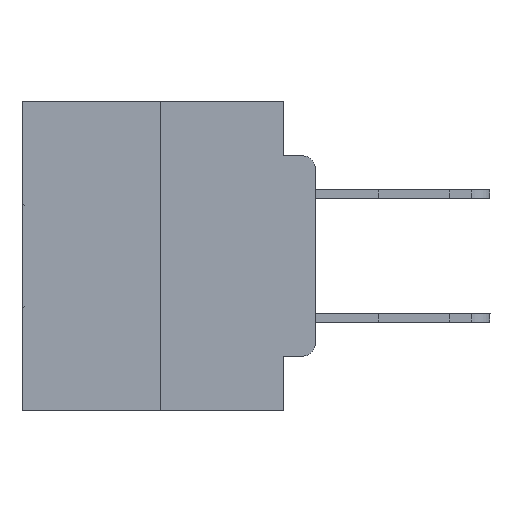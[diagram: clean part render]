
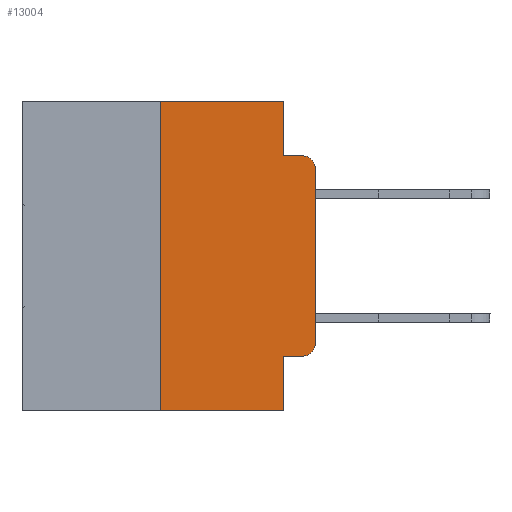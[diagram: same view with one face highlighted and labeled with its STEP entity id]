
A CAD part, left-side view. The second image highlights one B-rep face of the part: STEP entity #13004.
In plain terms, the highlighted planar face has unit normal (-1, 0, 0).
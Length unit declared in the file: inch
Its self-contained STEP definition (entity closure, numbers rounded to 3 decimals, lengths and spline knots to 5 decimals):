
#604 = EDGE_CURVE ( 'NONE', #9480, #17021, #27787, .T. ) ;
#773 = DIRECTION ( 'NONE',  ( 0., -1., 0. ) ) ;
#1050 = VERTEX_POINT ( 'NONE', #23095 ) ;
#1569 = ORIENTED_EDGE ( 'NONE', *, *, #604, .F. ) ;
#1609 = VECTOR ( 'NONE', #773, 39.37008 ) ;
#2639 = DIRECTION ( 'NONE',  ( 0., 0., -1. ) ) ;
#2685 = VECTOR ( 'NONE', #3333, 39.37008 ) ;
#3333 = DIRECTION ( 'NONE',  ( 0., 0., -1. ) ) ;
#3378 = CIRCLE ( 'NONE', #3551, 0.02 ) ;
#3551 = AXIS2_PLACEMENT_3D ( 'NONE', #14198, #12220, #28880 ) ;
#5192 = LINE ( 'NONE', #18729, #28688 ) ;
#5679 = DIRECTION ( 'NONE',  ( -1., 0., 0. ) ) ;
#5706 = CARTESIAN_POINT ( 'NONE',  ( 0., 0.051, 0. ) ) ;
#6138 = EDGE_CURVE ( 'NONE', #16923, #23357, #5192, .T. ) ;
#6221 = EDGE_CURVE ( 'NONE', #16923, #28515, #27536, .T. ) ;
#6909 = EDGE_CURVE ( 'NONE', #23357, #25650, #25981, .T. ) ;
#8230 = CIRCLE ( 'NONE', #27847, 0.02 ) ;
#8914 = VECTOR ( 'NONE', #18542, 39.37008 ) ;
#9053 = VERTEX_POINT ( 'NONE', #15930 ) ;
#9480 = VERTEX_POINT ( 'NONE', #10230 ) ;
#10230 = CARTESIAN_POINT ( 'NONE',  ( 0., 0.051, -0.0885 ) ) ;
#10297 = EDGE_CURVE ( 'NONE', #25650, #9480, #11986, .T. ) ;
#11095 = ORIENTED_EDGE ( 'NONE', *, *, #16214, .T. ) ;
#11140 = VECTOR ( 'NONE', #17852, 39.37008 ) ;
#11986 = LINE ( 'NONE', #5706, #2685 ) ;
#12096 = CARTESIAN_POINT ( 'NONE',  ( 0., 0.473, 0. ) ) ;
#12220 = DIRECTION ( 'NONE',  ( -1., 0., 0. ) ) ;
#12389 = DIRECTION ( 'NONE',  ( 1., 0., 0. ) ) ;
#12537 = VERTEX_POINT ( 'NONE', #24697 ) ;
#12599 = CARTESIAN_POINT ( 'NONE',  ( 0., 0.051, 0. ) ) ;
#12623 = LINE ( 'NONE', #17647, #11140 ) ;
#13004 = ADVANCED_FACE ( 'NONE', ( #19581 ), #17098, .F. ) ;
#13483 = CARTESIAN_POINT ( 'NONE',  ( 0., 0.051, 0. ) ) ;
#13714 = ORIENTED_EDGE ( 'NONE', *, *, #6909, .F. ) ;
#14068 = VECTOR ( 'NONE', #23597, 39.37008 ) ;
#14198 = CARTESIAN_POINT ( 'NONE',  ( 0., 0.02, -0.1085 ) ) ;
#14331 = EDGE_CURVE ( 'NONE', #9053, #1050, #20246, .T. ) ;
#15187 = DIRECTION ( 'NONE',  ( 0., -1., 0. ) ) ;
#15411 = EDGE_CURVE ( 'NONE', #1050, #12537, #8230, .T. ) ;
#15505 = CARTESIAN_POINT ( 'NONE',  ( 0., 0.051, -0.0885 ) ) ;
#15653 = ORIENTED_EDGE ( 'NONE', *, *, #27863, .F. ) ;
#15930 = CARTESIAN_POINT ( 'NONE',  ( 0., 0.051, -0.4115 ) ) ;
#16000 = DIRECTION ( 'NONE',  ( 0., 0., -1. ) ) ;
#16214 = EDGE_CURVE ( 'NONE', #21016, #17021, #3378, .T. ) ;
#16517 = CARTESIAN_POINT ( 'NONE',  ( 0., 0.473, 0. ) ) ;
#16923 = VERTEX_POINT ( 'NONE', #22197 ) ;
#17021 = VERTEX_POINT ( 'NONE', #29973 ) ;
#17098 = PLANE ( 'NONE',  #28214 ) ;
#17332 = CARTESIAN_POINT ( 'NONE',  ( 0., 0.051, -0.4115 ) ) ;
#17609 = CARTESIAN_POINT ( 'NONE',  ( 0., 0., -0.1085 ) ) ;
#17647 = CARTESIAN_POINT ( 'NONE',  ( 0., 0., 0. ) ) ;
#17852 = DIRECTION ( 'NONE',  ( 0., 0., 1. ) ) ;
#18068 = CARTESIAN_POINT ( 'NONE',  ( 0., 0.25, 0. ) ) ;
#18542 = DIRECTION ( 'NONE',  ( 0., -1., 0. ) ) ;
#18729 = CARTESIAN_POINT ( 'NONE',  ( 0., 0.25, 0. ) ) ;
#19176 = ORIENTED_EDGE ( 'NONE', *, *, #20363, .T. ) ;
#19581 = FACE_OUTER_BOUND ( 'NONE', #21613, .T. ) ;
#20246 = LINE ( 'NONE', #17332, #1609 ) ;
#20363 = EDGE_CURVE ( 'NONE', #12537, #21016, #12623, .T. ) ;
#21016 = VERTEX_POINT ( 'NONE', #17609 ) ;
#21325 = ORIENTED_EDGE ( 'NONE', *, *, #10297, .F. ) ;
#21470 = VECTOR ( 'NONE', #15187, 39.37008 ) ;
#21613 = EDGE_LOOP ( 'NONE', ( #19176, #11095, #1569, #21325, #13714, #30451, #22222, #15653, #27910, #24919 ) ) ;
#22197 = CARTESIAN_POINT ( 'NONE',  ( 0., 0.25, -0.5 ) ) ;
#22222 = ORIENTED_EDGE ( 'NONE', *, *, #6221, .T. ) ;
#23068 = VECTOR ( 'NONE', #16000, 39.37008 ) ;
#23095 = CARTESIAN_POINT ( 'NONE',  ( 0., 0.02, -0.4115 ) ) ;
#23357 = VERTEX_POINT ( 'NONE', #18068 ) ;
#23597 = DIRECTION ( 'NONE',  ( 0., -1., 0. ) ) ;
#24697 = CARTESIAN_POINT ( 'NONE',  ( 0., 0., -0.3915 ) ) ;
#24919 = ORIENTED_EDGE ( 'NONE', *, *, #15411, .T. ) ;
#25419 = CARTESIAN_POINT ( 'NONE',  ( 0., 0.051, -0.5 ) ) ;
#25650 = VERTEX_POINT ( 'NONE', #12599 ) ;
#25874 = DIRECTION ( 'NONE',  ( 0., 0., 1. ) ) ;
#25981 = LINE ( 'NONE', #16517, #14068 ) ;
#25991 = CARTESIAN_POINT ( 'NONE',  ( 0., 0.02, -0.3915 ) ) ;
#27536 = LINE ( 'NONE', #28514, #8914 ) ;
#27787 = LINE ( 'NONE', #15505, #21470 ) ;
#27847 = AXIS2_PLACEMENT_3D ( 'NONE', #25991, #5679, #30701 ) ;
#27863 = EDGE_CURVE ( 'NONE', #9053, #28515, #28637, .T. ) ;
#27910 = ORIENTED_EDGE ( 'NONE', *, *, #14331, .T. ) ;
#28214 = AXIS2_PLACEMENT_3D ( 'NONE', #12096, #12389, #2639 ) ;
#28514 = CARTESIAN_POINT ( 'NONE',  ( 0., 0.473, -0.5 ) ) ;
#28515 = VERTEX_POINT ( 'NONE', #25419 ) ;
#28637 = LINE ( 'NONE', #13483, #23068 ) ;
#28688 = VECTOR ( 'NONE', #25874, 39.37008 ) ;
#28880 = DIRECTION ( 'NONE',  ( 0., 0., -1. ) ) ;
#29973 = CARTESIAN_POINT ( 'NONE',  ( 0., 0.02, -0.0885 ) ) ;
#30451 = ORIENTED_EDGE ( 'NONE', *, *, #6138, .F. ) ;
#30701 = DIRECTION ( 'NONE',  ( 0., 0., -1. ) ) ;
